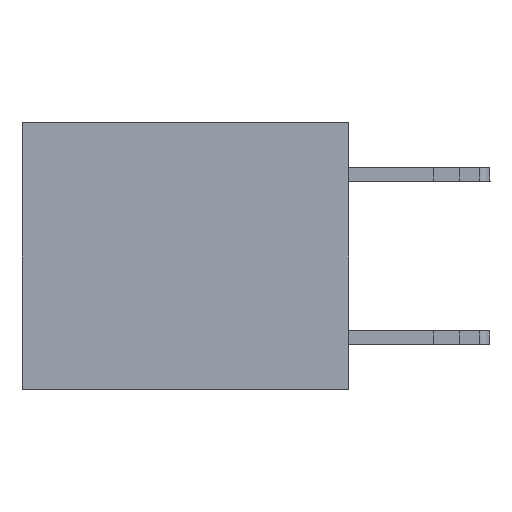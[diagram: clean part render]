
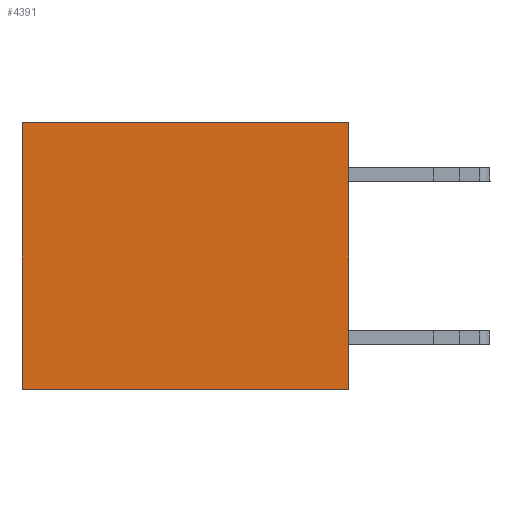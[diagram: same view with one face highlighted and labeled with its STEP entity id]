
A CAD part, left-side view. The second image highlights one B-rep face of the part: STEP entity #4391.
In plain terms, the highlighted planar face has unit normal (-1, 0, 0).
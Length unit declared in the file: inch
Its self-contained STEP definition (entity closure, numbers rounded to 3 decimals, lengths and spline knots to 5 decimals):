
#323 = VERTEX_POINT ( 'NONE', #16002 ) ;
#465 = CARTESIAN_POINT ( 'NONE',  ( 0.3165, 0., -0.49 ) ) ;
#587 = CARTESIAN_POINT ( 'NONE',  ( 0.3165, 0.6, -0.49 ) ) ;
#727 = LINE ( 'NONE', #11745, #4785 ) ;
#1047 = EDGE_CURVE ( 'NONE', #11928, #14514, #15147, .T. ) ;
#1307 = DIRECTION ( 'NONE',  ( 0., 0., -1. ) ) ;
#1308 = PLANE ( 'NONE',  #15306 ) ;
#1472 = CARTESIAN_POINT ( 'NONE',  ( 0.3165, 0., -0.49 ) ) ;
#2371 = DIRECTION ( 'NONE',  ( 0., 1., 0. ) ) ;
#4391 = ADVANCED_FACE ( 'NONE', ( #7179 ), #1308, .F. ) ;
#4785 = VECTOR ( 'NONE', #8511, 39.37008 ) ;
#6561 = VERTEX_POINT ( 'NONE', #19516 ) ;
#7179 = FACE_OUTER_BOUND ( 'NONE', #14949, .T. ) ;
#7326 = VECTOR ( 'NONE', #2371, 39.37008 ) ;
#7924 = DIRECTION ( 'NONE',  ( 1., 0., 0. ) ) ;
#8350 = EDGE_CURVE ( 'NONE', #323, #6561, #727, .T. ) ;
#8511 = DIRECTION ( 'NONE',  ( 0., 1., 0. ) ) ;
#9028 = CARTESIAN_POINT ( 'NONE',  ( 0.3165, 0.6, -0.49 ) ) ;
#9064 = ORIENTED_EDGE ( 'NONE', *, *, #8350, .T. ) ;
#10118 = VECTOR ( 'NONE', #20626, 39.37008 ) ;
#10535 = CARTESIAN_POINT ( 'NONE',  ( 0.3165, 0., -0.49 ) ) ;
#10891 = LINE ( 'NONE', #9028, #10118 ) ;
#11037 = CARTESIAN_POINT ( 'NONE',  ( 0.3165, 0., -0.49 ) ) ;
#11327 = ORIENTED_EDGE ( 'NONE', *, *, #16297, .T. ) ;
#11745 = CARTESIAN_POINT ( 'NONE',  ( 0.3165, 0., 0. ) ) ;
#11928 = VERTEX_POINT ( 'NONE', #1472 ) ;
#14514 = VERTEX_POINT ( 'NONE', #587 ) ;
#14949 = EDGE_LOOP ( 'NONE', ( #11327, #15492, #19295, #9064 ) ) ;
#15147 = LINE ( 'NONE', #10535, #7326 ) ;
#15306 = AXIS2_PLACEMENT_3D ( 'NONE', #11037, #7924, #18933 ) ;
#15443 = VECTOR ( 'NONE', #1307, 39.37008 ) ;
#15492 = ORIENTED_EDGE ( 'NONE', *, *, #1047, .F. ) ;
#16002 = CARTESIAN_POINT ( 'NONE',  ( 0.3165, 0., 0. ) ) ;
#16297 = EDGE_CURVE ( 'NONE', #6561, #14514, #10891, .T. ) ;
#17214 = LINE ( 'NONE', #465, #15443 ) ;
#18933 = DIRECTION ( 'NONE',  ( 0., 0., -1. ) ) ;
#19295 = ORIENTED_EDGE ( 'NONE', *, *, #20567, .F. ) ;
#19516 = CARTESIAN_POINT ( 'NONE',  ( 0.3165, 0.6, 0. ) ) ;
#20567 = EDGE_CURVE ( 'NONE', #323, #11928, #17214, .T. ) ;
#20626 = DIRECTION ( 'NONE',  ( 0., 0., -1. ) ) ;
